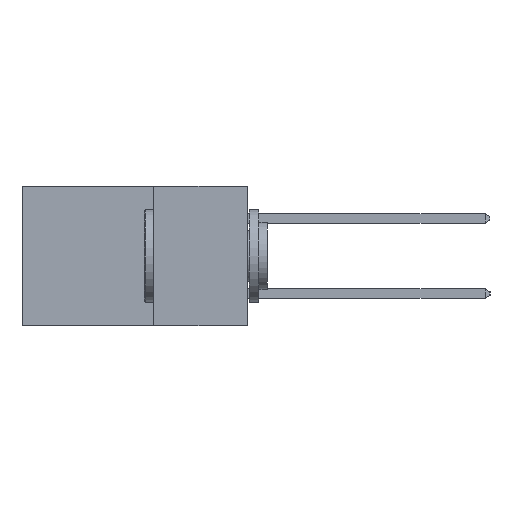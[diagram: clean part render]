
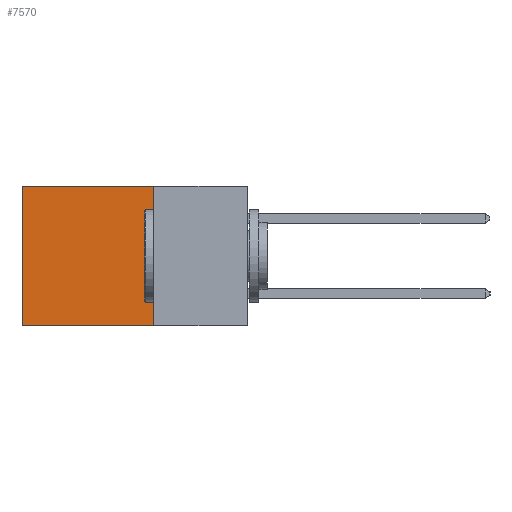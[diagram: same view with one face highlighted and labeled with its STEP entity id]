
A CAD part, left-side view. The second image highlights one B-rep face of the part: STEP entity #7570.
In plain terms, the highlighted planar face has unit normal (-1, 0, 0).
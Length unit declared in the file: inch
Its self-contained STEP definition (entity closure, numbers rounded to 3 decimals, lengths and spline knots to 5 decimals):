
#131 = PLANE ( 'NONE',  #15394 ) ;
#1072 = DIRECTION ( 'NONE',  ( 0., 0., -1. ) ) ;
#1128 = CARTESIAN_POINT ( 'NONE',  ( 0.2615, 0.6, -0.37 ) ) ;
#1632 = CARTESIAN_POINT ( 'NONE',  ( 0.2615, 0.25, 0. ) ) ;
#1669 = DIRECTION ( 'NONE',  ( 1., 0., 0. ) ) ;
#1855 = FACE_OUTER_BOUND ( 'NONE', #15555, .T. ) ;
#2465 = VERTEX_POINT ( 'NONE', #9110 ) ;
#2678 = LINE ( 'NONE', #11690, #6117 ) ;
#2810 = CARTESIAN_POINT ( 'NONE',  ( 0.2615, 0.6, 0. ) ) ;
#3646 = VERTEX_POINT ( 'NONE', #2810 ) ;
#4865 = CARTESIAN_POINT ( 'NONE',  ( 0.2615, 0.25, 0. ) ) ;
#5236 = ORIENTED_EDGE ( 'NONE', *, *, #18417, .F. ) ;
#6117 = VECTOR ( 'NONE', #15797, 39.37008 ) ;
#6336 = DIRECTION ( 'NONE',  ( 0., 1., 0. ) ) ;
#7281 = ORIENTED_EDGE ( 'NONE', *, *, #14117, .T. ) ;
#7570 = ADVANCED_FACE ( 'NONE', ( #1855 ), #131, .F. ) ;
#8205 = DIRECTION ( 'NONE',  ( 0., 0., -1. ) ) ;
#8956 = CARTESIAN_POINT ( 'NONE',  ( 0.2615, 0.25, -0.37 ) ) ;
#9110 = CARTESIAN_POINT ( 'NONE',  ( 0.2615, 0.25, -0.37 ) ) ;
#9331 = VECTOR ( 'NONE', #1072, 39.37008 ) ;
#9584 = VECTOR ( 'NONE', #8205, 39.37008 ) ;
#10542 = EDGE_CURVE ( 'NONE', #2465, #12486, #2678, .T. ) ;
#11690 = CARTESIAN_POINT ( 'NONE',  ( 0.2615, 0.25, -0.37 ) ) ;
#11693 = CARTESIAN_POINT ( 'NONE',  ( 0.2615, 0.6, -0.37 ) ) ;
#11785 = DIRECTION ( 'NONE',  ( 0., 0., -1. ) ) ;
#12413 = CARTESIAN_POINT ( 'NONE',  ( 0.2615, 0.25, -0.37 ) ) ;
#12486 = VERTEX_POINT ( 'NONE', #11693 ) ;
#12971 = LINE ( 'NONE', #4865, #16638 ) ;
#13276 = LINE ( 'NONE', #12413, #9584 ) ;
#14117 = EDGE_CURVE ( 'NONE', #3646, #12486, #16699, .T. ) ;
#15060 = VERTEX_POINT ( 'NONE', #1632 ) ;
#15394 = AXIS2_PLACEMENT_3D ( 'NONE', #8956, #1669, #11785 ) ;
#15555 = EDGE_LOOP ( 'NONE', ( #7281, #17989, #5236, #16158 ) ) ;
#15797 = DIRECTION ( 'NONE',  ( 0., 1., 0. ) ) ;
#15849 = EDGE_CURVE ( 'NONE', #15060, #3646, #12971, .T. ) ;
#16158 = ORIENTED_EDGE ( 'NONE', *, *, #15849, .T. ) ;
#16638 = VECTOR ( 'NONE', #6336, 39.37008 ) ;
#16699 = LINE ( 'NONE', #1128, #9331 ) ;
#17989 = ORIENTED_EDGE ( 'NONE', *, *, #10542, .F. ) ;
#18417 = EDGE_CURVE ( 'NONE', #15060, #2465, #13276, .T. ) ;
